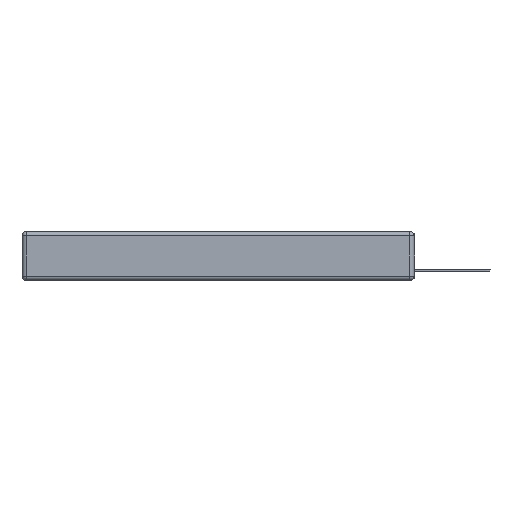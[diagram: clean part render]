
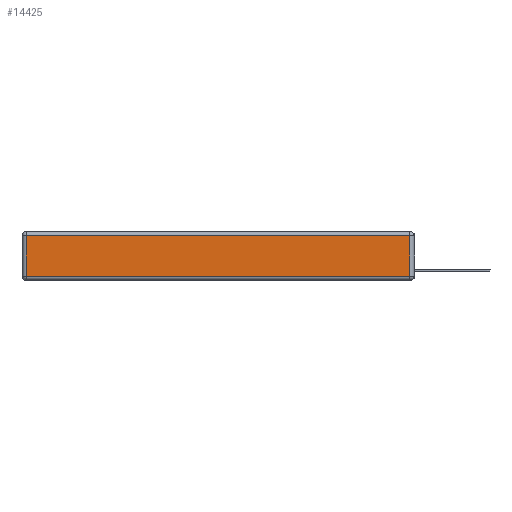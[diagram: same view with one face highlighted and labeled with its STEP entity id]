
A CAD part, left-side view. The second image highlights one B-rep face of the part: STEP entity #14425.
In plain terms, the highlighted planar face has unit normal (-1, 0, 0).
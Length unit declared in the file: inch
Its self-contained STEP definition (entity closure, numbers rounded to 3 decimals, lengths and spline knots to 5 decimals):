
#418 = DIRECTION ( 'NONE',  ( 0., 0., 1. ) ) ;
#1712 = CARTESIAN_POINT ( 'NONE',  ( 0., 0., -0.313 ) ) ;
#1800 = FACE_OUTER_BOUND ( 'NONE', #11641, .T. ) ;
#2277 = ORIENTED_EDGE ( 'NONE', *, *, #6805, .T. ) ;
#2319 = DIRECTION ( 'NONE',  ( 0., 0., 1. ) ) ;
#2320 = LINE ( 'NONE', #5525, #7631 ) ;
#2463 = VERTEX_POINT ( 'NONE', #10694 ) ;
#2546 = VECTOR ( 'NONE', #418, 39.37008 ) ;
#2933 = LINE ( 'NONE', #9793, #2546 ) ;
#3131 = DIRECTION ( 'NONE',  ( 0., 1., 0. ) ) ;
#3394 = VERTEX_POINT ( 'NONE', #7005 ) ;
#3871 = VERTEX_POINT ( 'NONE', #6529 ) ;
#4378 = ORIENTED_EDGE ( 'NONE', *, *, #12441, .T. ) ;
#5329 = AXIS2_PLACEMENT_3D ( 'NONE', #10768, #6056, #2319 ) ;
#5525 = CARTESIAN_POINT ( 'NONE',  ( 0., 2.75, -0.03 ) ) ;
#6056 = DIRECTION ( 'NONE',  ( -1., 0., 0. ) ) ;
#6529 = CARTESIAN_POINT ( 'NONE',  ( 0., 2.72, -0.03 ) ) ;
#6805 = EDGE_CURVE ( 'NONE', #2463, #3394, #9214, .T. ) ;
#6817 = VECTOR ( 'NONE', #7849, 39.37008 ) ;
#7005 = CARTESIAN_POINT ( 'NONE',  ( 0., 0.03, -0.313 ) ) ;
#7015 = ORIENTED_EDGE ( 'NONE', *, *, #9222, .T. ) ;
#7631 = VECTOR ( 'NONE', #3131, 39.37008 ) ;
#7849 = DIRECTION ( 'NONE',  ( 0., 0., -1. ) ) ;
#9206 = VERTEX_POINT ( 'NONE', #10077 ) ;
#9214 = LINE ( 'NONE', #1712, #14726 ) ;
#9222 = EDGE_CURVE ( 'NONE', #9206, #3871, #2320, .T. ) ;
#9575 = PLANE ( 'NONE',  #5329 ) ;
#9793 = CARTESIAN_POINT ( 'NONE',  ( 0., 0.03, -0.343 ) ) ;
#9983 = LINE ( 'NONE', #14912, #6817 ) ;
#10077 = CARTESIAN_POINT ( 'NONE',  ( 0., 0.03, -0.03 ) ) ;
#10694 = CARTESIAN_POINT ( 'NONE',  ( 0., 2.72, -0.313 ) ) ;
#10768 = CARTESIAN_POINT ( 'NONE',  ( 0., 0., -0.343 ) ) ;
#11641 = EDGE_LOOP ( 'NONE', ( #2277, #15079, #7015, #4378 ) ) ;
#12366 = DIRECTION ( 'NONE',  ( 0., -1., 0. ) ) ;
#12441 = EDGE_CURVE ( 'NONE', #3871, #2463, #9983, .T. ) ;
#14150 = EDGE_CURVE ( 'NONE', #3394, #9206, #2933, .T. ) ;
#14425 = ADVANCED_FACE ( 'NONE', ( #1800 ), #9575, .T. ) ;
#14726 = VECTOR ( 'NONE', #12366, 39.37008 ) ;
#14912 = CARTESIAN_POINT ( 'NONE',  ( 0., 2.72, -0.343 ) ) ;
#15079 = ORIENTED_EDGE ( 'NONE', *, *, #14150, .T. ) ;
